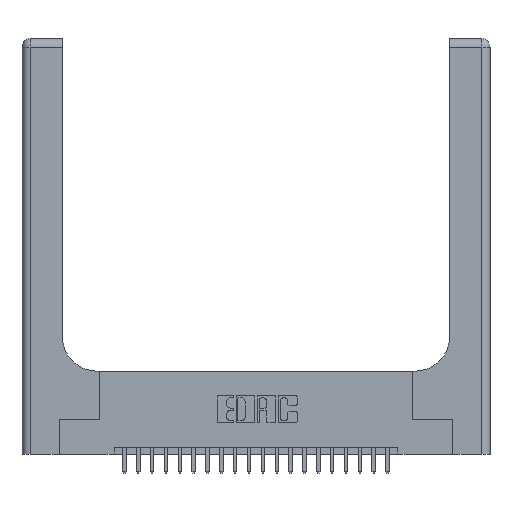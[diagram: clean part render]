
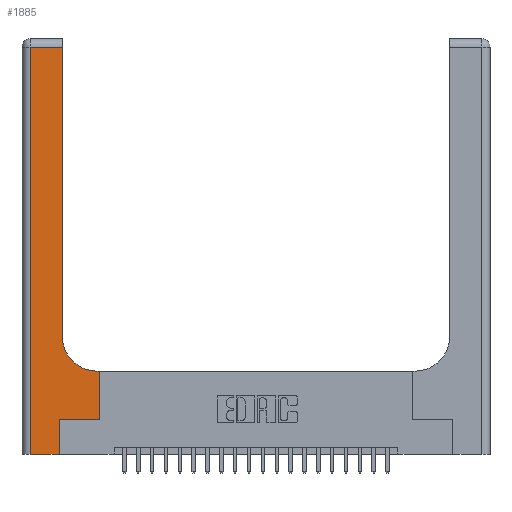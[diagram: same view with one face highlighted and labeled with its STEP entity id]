
A CAD part, top view. The second image highlights one B-rep face of the part: STEP entity #1885.
In plain terms, the highlighted planar face has unit normal (0, 0, 1).
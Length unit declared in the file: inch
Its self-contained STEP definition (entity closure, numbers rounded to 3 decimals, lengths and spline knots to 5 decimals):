
#53 = CARTESIAN_POINT ( 'NONE',  ( 0.06, 2.94, 0.37 ) ) ;
#676 = CARTESIAN_POINT ( 'NONE',  ( 0.06, 0., 0.37 ) ) ;
#1131 = EDGE_CURVE ( 'NONE', #11140, #6456, #23781, .T. ) ;
#1461 = EDGE_LOOP ( 'NONE', ( #5052, #7503, #13633, #7387, #14362, #5526, #16034, #3964, #17615 ) ) ;
#1885 = ADVANCED_FACE ( 'NONE', ( #3535 ), #10052, .F. ) ;
#2175 = CARTESIAN_POINT ( 'NONE',  ( 0.5415, 0.85, 0.37 ) ) ;
#2568 = VECTOR ( 'NONE', #11191, 39.37008 ) ;
#3019 = VECTOR ( 'NONE', #12797, 39.37008 ) ;
#3535 = FACE_OUTER_BOUND ( 'NONE', #1461, .T. ) ;
#3743 = CARTESIAN_POINT ( 'NONE',  ( 0.5585, 0.25, 0.37 ) ) ;
#3964 = ORIENTED_EDGE ( 'NONE', *, *, #12428, .T. ) ;
#4861 = VERTEX_POINT ( 'NONE', #676 ) ;
#5052 = ORIENTED_EDGE ( 'NONE', *, *, #23080, .T. ) ;
#5494 = CARTESIAN_POINT ( 'NONE',  ( 0., 0., 0.37 ) ) ;
#5526 = ORIENTED_EDGE ( 'NONE', *, *, #11294, .T. ) ;
#5972 = DIRECTION ( 'NONE',  ( 0., 0., -1. ) ) ;
#6376 = EDGE_CURVE ( 'NONE', #15165, #19187, #15650, .T. ) ;
#6456 = VERTEX_POINT ( 'NONE', #15988 ) ;
#6506 = VERTEX_POINT ( 'NONE', #19674 ) ;
#6932 = EDGE_CURVE ( 'NONE', #19773, #4861, #11028, .T. ) ;
#7141 = DIRECTION ( 'NONE',  ( 0., 1., 0. ) ) ;
#7387 = ORIENTED_EDGE ( 'NONE', *, *, #13315, .T. ) ;
#7503 = ORIENTED_EDGE ( 'NONE', *, *, #11603, .T. ) ;
#7886 = LINE ( 'NONE', #21957, #11949 ) ;
#8343 = DIRECTION ( 'NONE',  ( 0., 0., -1. ) ) ;
#8697 = VECTOR ( 'NONE', #18871, 39.37008 ) ;
#9206 = VECTOR ( 'NONE', #10730, 39.37008 ) ;
#9237 = AXIS2_PLACEMENT_3D ( 'NONE', #2175, #5972, #15158 ) ;
#9865 = LINE ( 'NONE', #10259, #14233 ) ;
#10052 = PLANE ( 'NONE',  #12904 ) ;
#10259 = CARTESIAN_POINT ( 'NONE',  ( 0.2915, 3., 0.37 ) ) ;
#10706 = VECTOR ( 'NONE', #18691, 39.37008 ) ;
#10730 = DIRECTION ( 'NONE',  ( -1., 0., 0. ) ) ;
#10821 = DIRECTION ( 'NONE',  ( -1., 0., 0. ) ) ;
#10937 = CARTESIAN_POINT ( 'NONE',  ( 0.2915, 2.94, 0.37 ) ) ;
#11028 = LINE ( 'NONE', #15511, #8697 ) ;
#11140 = VERTEX_POINT ( 'NONE', #3743 ) ;
#11191 = DIRECTION ( 'NONE',  ( 1., 0., 0. ) ) ;
#11294 = EDGE_CURVE ( 'NONE', #6506, #11140, #13870, .T. ) ;
#11603 = EDGE_CURVE ( 'NONE', #14196, #19773, #17578, .T. ) ;
#11949 = VECTOR ( 'NONE', #7141, 39.37008 ) ;
#12312 = CARTESIAN_POINT ( 'NONE',  ( 0., 3., 0.37 ) ) ;
#12428 = EDGE_CURVE ( 'NONE', #6456, #15165, #22449, .T. ) ;
#12797 = DIRECTION ( 'NONE',  ( 0., 1., 0. ) ) ;
#12904 = AXIS2_PLACEMENT_3D ( 'NONE', #12312, #8343, #23769 ) ;
#13315 = EDGE_CURVE ( 'NONE', #4861, #19768, #23623, .T. ) ;
#13338 = CARTESIAN_POINT ( 'NONE',  ( 0.269, 0., 0.37 ) ) ;
#13633 = ORIENTED_EDGE ( 'NONE', *, *, #6932, .T. ) ;
#13870 = LINE ( 'NONE', #15025, #10706 ) ;
#14196 = VERTEX_POINT ( 'NONE', #10937 ) ;
#14233 = VECTOR ( 'NONE', #15661, 39.37008 ) ;
#14362 = ORIENTED_EDGE ( 'NONE', *, *, #15784, .T. ) ;
#15025 = CARTESIAN_POINT ( 'NONE',  ( 0.269, 0.25, 0.37 ) ) ;
#15158 = DIRECTION ( 'NONE',  ( 1., 0., 0. ) ) ;
#15165 = VERTEX_POINT ( 'NONE', #15783 ) ;
#15511 = CARTESIAN_POINT ( 'NONE',  ( 0.06, 3., 0.37 ) ) ;
#15650 = CIRCLE ( 'NONE', #9237, 0.25 ) ;
#15661 = DIRECTION ( 'NONE',  ( 0., 1., 0. ) ) ;
#15783 = CARTESIAN_POINT ( 'NONE',  ( 0.5415, 0.6, 0.37 ) ) ;
#15784 = EDGE_CURVE ( 'NONE', #19768, #6506, #7886, .T. ) ;
#15988 = CARTESIAN_POINT ( 'NONE',  ( 0.5585, 0.6, 0.37 ) ) ;
#16034 = ORIENTED_EDGE ( 'NONE', *, *, #1131, .T. ) ;
#17289 = CARTESIAN_POINT ( 'NONE',  ( 0.2915, 0.85, 0.37 ) ) ;
#17578 = LINE ( 'NONE', #17883, #9206 ) ;
#17615 = ORIENTED_EDGE ( 'NONE', *, *, #6376, .T. ) ;
#17883 = CARTESIAN_POINT ( 'NONE',  ( 0., 2.94, 0.37 ) ) ;
#18691 = DIRECTION ( 'NONE',  ( 1., 0., 0. ) ) ;
#18871 = DIRECTION ( 'NONE',  ( 0., -1., 0. ) ) ;
#19187 = VERTEX_POINT ( 'NONE', #17289 ) ;
#19674 = CARTESIAN_POINT ( 'NONE',  ( 0.269, 0.25, 0.37 ) ) ;
#19768 = VERTEX_POINT ( 'NONE', #13338 ) ;
#19773 = VERTEX_POINT ( 'NONE', #53 ) ;
#19815 = CARTESIAN_POINT ( 'NONE',  ( 0.2915, 0.6, 0.37 ) ) ;
#20208 = CARTESIAN_POINT ( 'NONE',  ( 0.5585, 0.25, 0.37 ) ) ;
#21957 = CARTESIAN_POINT ( 'NONE',  ( 0.269, 0., 0.37 ) ) ;
#22449 = LINE ( 'NONE', #19815, #23020 ) ;
#23020 = VECTOR ( 'NONE', #10821, 39.37008 ) ;
#23080 = EDGE_CURVE ( 'NONE', #19187, #14196, #9865, .T. ) ;
#23623 = LINE ( 'NONE', #5494, #2568 ) ;
#23769 = DIRECTION ( 'NONE',  ( -1., 0., 0. ) ) ;
#23781 = LINE ( 'NONE', #20208, #3019 ) ;
